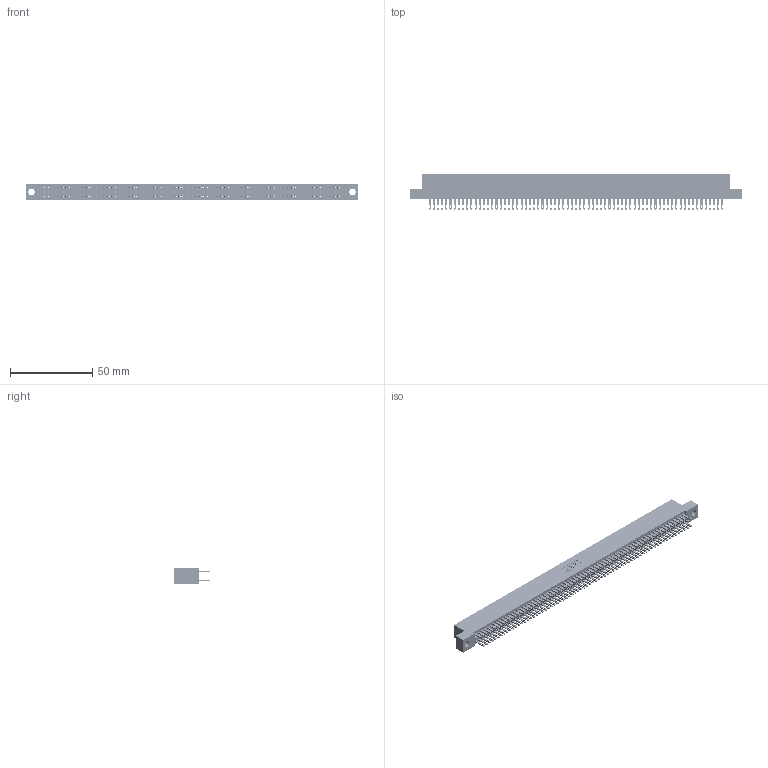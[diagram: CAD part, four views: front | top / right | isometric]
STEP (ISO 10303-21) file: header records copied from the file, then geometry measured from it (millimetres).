
FILE_DESCRIPTION (( 'STEP AP203' ), '1' );
FILE_NAME ('345-142-500-204.STEP', '2018-10-21T02:51:14', ( '' ), ( '' ), 'SwSTEP 2.0', 'SolidWorks 2016', '' );
FILE_SCHEMA (( 'CONFIG_CONTROL_DESIGN' ));
Length unit declared in the file: inch
Products named in the file (3): 345-142-500-204; 345-292-001_345-293-100; 345 Part_Flush Mounting Lugs - 0.156 Dia-TH
Assembly tree (143 placements, depth 2):
  345-142-500-204
    345 Part_Flush Mounting Lugs - 0.156 Dia-TH
    345-292-001_345-293-100  x142
Bounding box: 201.55 x 21.51 x 9.4 mm (x, y, z)
Volume: 20193.9 mm3; surface area: 31675.2 mm2
Topology: 143 solids, 143 shells, 6658 faces, 20363 edges, 13574 vertices
Faces by surface type: plane 3914, cylinder 2744
Entity records: 51737 total; most frequent: CARTESIAN_POINT 8644, ORIENTED_EDGE 8578, DIRECTION 7589, EDGE_CURVE 4289, LINE 3869, VECTOR 3869, VERTEX_POINT 2858, AXIS2_PLACEMENT_3D 1860
